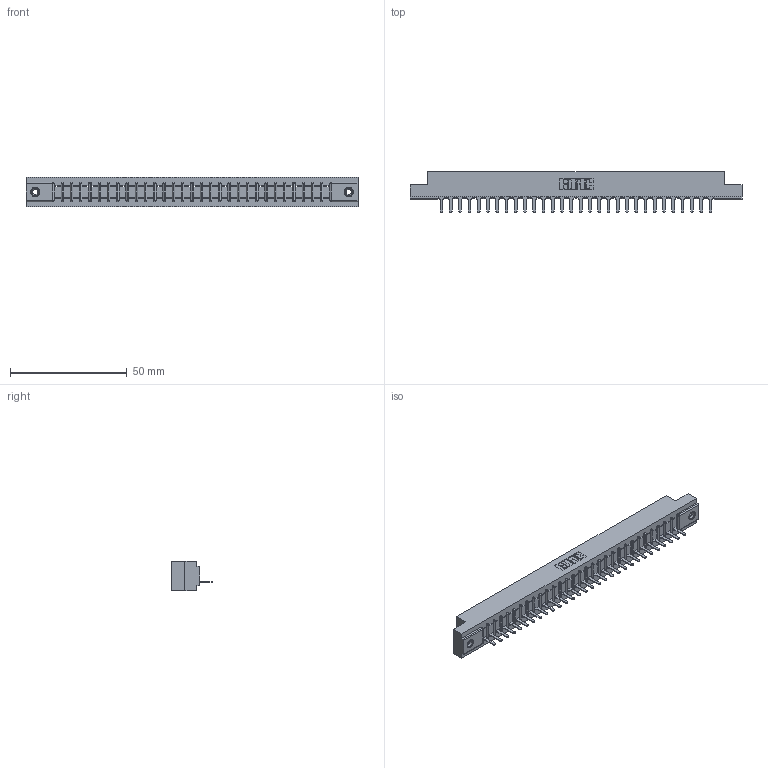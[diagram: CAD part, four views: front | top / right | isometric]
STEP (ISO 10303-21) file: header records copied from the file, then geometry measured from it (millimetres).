
FILE_DESCRIPTION (( 'STEP AP203' ), '1' );
FILE_NAME ('357-030-425-108.STEP', '2020-10-02T00:25:34', ( '' ), ( '' ), 'SwSTEP 2.0', 'SolidWorks 2020', '' );
FILE_SCHEMA (( 'CONFIG_CONTROL_DESIGN' ));
Length unit declared in the file: inch
Products named in the file (4): 357-030-425-108; 307-290-001_525; 345-250-001_345-250-003-102; 307 Part_.156 Dia Mounting Holes
Assembly tree (33 placements, depth 2):
  357-030-425-108
    307 Part_.156 Dia Mounting Holes
    307-290-001_525  x30
    345-250-001_345-250-003-102  x2
Bounding box: 141.88 x 17.42 x 12.7 mm (x, y, z)
Volume: 14631.1 mm3; surface area: 15187.6 mm2
Topology: 33 solids, 33 shells, 1889 faces, 5319 edges, 3414 vertices
Faces by surface type: plane 1212, cylinder 599, sphere 62, cone 12, torus 4
Entity records: 28351 total; most frequent: CARTESIAN_POINT 4751, ORIENTED_EDGE 4730, DIRECTION 4637, EDGE_CURVE 2365, VECTOR 1809, LINE 1809, VERTEX_POINT 1528, AXIS2_PLACEMENT_3D 1414
